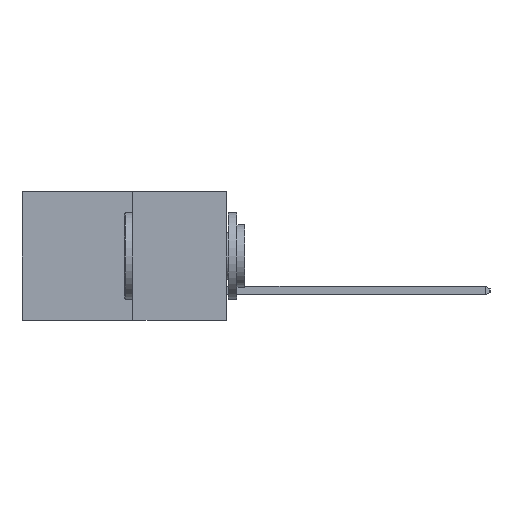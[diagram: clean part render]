
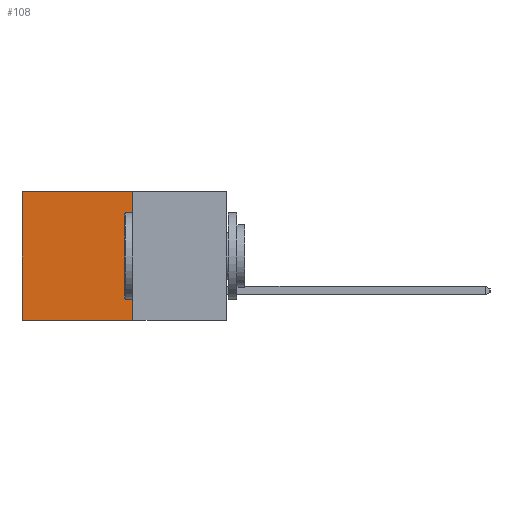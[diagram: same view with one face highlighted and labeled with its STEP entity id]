
A CAD part, left-side view. The second image highlights one B-rep face of the part: STEP entity #108.
In plain terms, the highlighted planar face has unit normal (-1, 0, 0).
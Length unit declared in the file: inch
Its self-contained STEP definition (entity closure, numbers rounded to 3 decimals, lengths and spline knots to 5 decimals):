
#108 = ADVANCED_FACE ( 'NONE', ( #2132 ), #7661, .F. ) ;
#477 = CARTESIAN_POINT ( 'NONE',  ( 0.277, 0.59, -0.37 ) ) ;
#554 = VECTOR ( 'NONE', #3550, 39.37008 ) ;
#578 = EDGE_CURVE ( 'NONE', #7220, #9922, #10224, .T. ) ;
#984 = DIRECTION ( 'NONE',  ( 0., 1., 0. ) ) ;
#1046 = EDGE_LOOP ( 'NONE', ( #10588, #9557, #10348, #5477 ) ) ;
#1697 = DIRECTION ( 'NONE',  ( 0., 1., 0. ) ) ;
#1718 = LINE ( 'NONE', #6676, #10112 ) ;
#2132 = FACE_OUTER_BOUND ( 'NONE', #1046, .T. ) ;
#2332 = VERTEX_POINT ( 'NONE', #477 ) ;
#2380 = CARTESIAN_POINT ( 'NONE',  ( 0.277, 0.27, -0.37 ) ) ;
#2700 = CARTESIAN_POINT ( 'NONE',  ( 0.277, 0.59, 0. ) ) ;
#2727 = VERTEX_POINT ( 'NONE', #2380 ) ;
#2833 = DIRECTION ( 'NONE',  ( 0., 0., -1. ) ) ;
#3508 = CARTESIAN_POINT ( 'NONE',  ( 0.277, 0.59, -0.37 ) ) ;
#3550 = DIRECTION ( 'NONE',  ( 0., 0., -1. ) ) ;
#4106 = CARTESIAN_POINT ( 'NONE',  ( 0.277, 0.27, 0. ) ) ;
#4335 = VECTOR ( 'NONE', #5213, 39.37008 ) ;
#4630 = CARTESIAN_POINT ( 'NONE',  ( 0.277, 0.27, -0.37 ) ) ;
#5213 = DIRECTION ( 'NONE',  ( 0., 0., -1. ) ) ;
#5477 = ORIENTED_EDGE ( 'NONE', *, *, #578, .T. ) ;
#6054 = CARTESIAN_POINT ( 'NONE',  ( 0.277, 0.27, -0.37 ) ) ;
#6267 = CARTESIAN_POINT ( 'NONE',  ( 0.277, 0.27, 0. ) ) ;
#6676 = CARTESIAN_POINT ( 'NONE',  ( 0.277, 0.27, -0.37 ) ) ;
#6766 = EDGE_CURVE ( 'NONE', #7220, #2727, #7513, .T. ) ;
#6771 = DIRECTION ( 'NONE',  ( 1., 0., 0. ) ) ;
#6815 = VECTOR ( 'NONE', #984, 39.37008 ) ;
#6830 = LINE ( 'NONE', #3508, #4335 ) ;
#7220 = VERTEX_POINT ( 'NONE', #4106 ) ;
#7513 = LINE ( 'NONE', #6054, #554 ) ;
#7647 = AXIS2_PLACEMENT_3D ( 'NONE', #4630, #6771, #2833 ) ;
#7661 = PLANE ( 'NONE',  #7647 ) ;
#8612 = EDGE_CURVE ( 'NONE', #9922, #2332, #6830, .T. ) ;
#9557 = ORIENTED_EDGE ( 'NONE', *, *, #10429, .F. ) ;
#9922 = VERTEX_POINT ( 'NONE', #2700 ) ;
#10112 = VECTOR ( 'NONE', #1697, 39.37008 ) ;
#10224 = LINE ( 'NONE', #6267, #6815 ) ;
#10348 = ORIENTED_EDGE ( 'NONE', *, *, #6766, .F. ) ;
#10429 = EDGE_CURVE ( 'NONE', #2727, #2332, #1718, .T. ) ;
#10588 = ORIENTED_EDGE ( 'NONE', *, *, #8612, .T. ) ;
